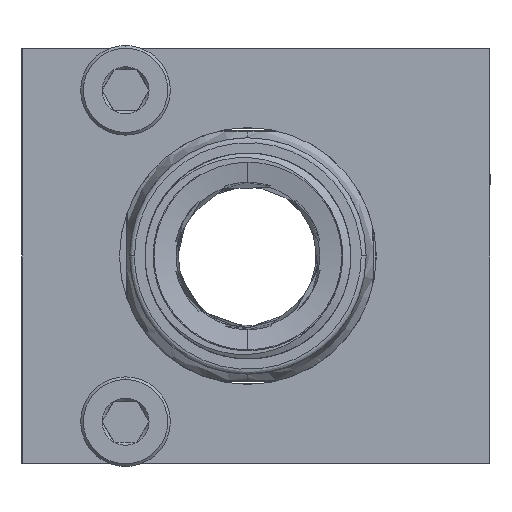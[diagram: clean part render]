
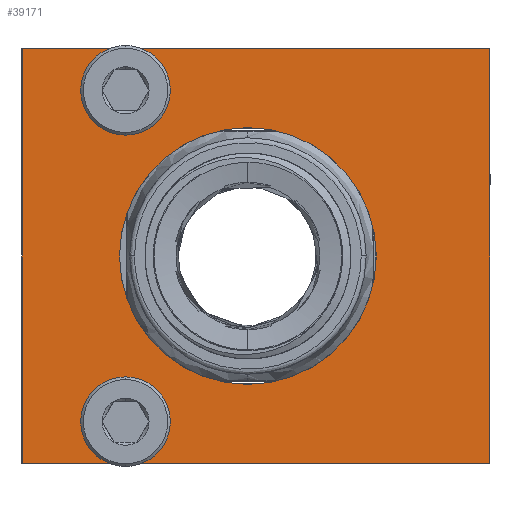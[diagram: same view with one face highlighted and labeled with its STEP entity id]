
A CAD part, left-side view. The second image highlights one B-rep face of the part: STEP entity #39171.
In plain terms, the highlighted face is planar.
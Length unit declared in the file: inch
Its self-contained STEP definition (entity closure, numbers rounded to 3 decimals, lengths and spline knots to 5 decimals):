
#398 = CARTESIAN_POINT ( 'NONE',  ( 0.1, -0.25, 0. ) ) ;
#2111 = CIRCLE ( 'NONE', #46787, 0.06693 ) ;
#2180 = CARTESIAN_POINT ( 'NONE',  ( 0., 0., 0. ) ) ;
#2478 = CARTESIAN_POINT ( 'NONE',  ( 0., -1.13, 0. ) ) ;
#2892 = CARTESIAN_POINT ( 'NONE',  ( 0.83307, -0.25, 0. ) ) ;
#3965 = CARTESIAN_POINT ( 'NONE',  ( 0., 0., 0. ) ) ;
#5410 = CARTESIAN_POINT ( 'NONE',  ( 0.03307, -0.25, 0. ) ) ;
#6128 = ORIENTED_EDGE ( 'NONE', *, *, #40474, .F. ) ;
#6226 = CARTESIAN_POINT ( 'NONE',  ( 1., 0., 0. ) ) ;
#8245 = VERTEX_POINT ( 'NONE', #2478 ) ;
#8386 = DIRECTION ( 'NONE',  ( 1., 0., 0. ) ) ;
#8398 = LINE ( 'NONE', #37738, #50243 ) ;
#8513 = CIRCLE ( 'NONE', #46215, 0.31 ) ;
#8878 = ORIENTED_EDGE ( 'NONE', *, *, #20147, .F. ) ;
#9260 = CARTESIAN_POINT ( 'NONE',  ( 0., -1.13, 0. ) ) ;
#9750 = CIRCLE ( 'NONE', #53628, 0.06693 ) ;
#10035 = VERTEX_POINT ( 'NONE', #11764 ) ;
#11414 = CARTESIAN_POINT ( 'NONE',  ( 0.5, -0.5454, 0. ) ) ;
#11764 = CARTESIAN_POINT ( 'NONE',  ( 0.19, -0.5454, 0. ) ) ;
#12238 = DIRECTION ( 'NONE',  ( 0., 0., 1. ) ) ;
#13380 = EDGE_CURVE ( 'NONE', #33789, #44122, #49512, .T. ) ;
#13901 = CARTESIAN_POINT ( 'NONE',  ( 0., 0., 0. ) ) ;
#14447 = LINE ( 'NONE', #13901, #34724 ) ;
#16477 = CARTESIAN_POINT ( 'NONE',  ( 0.9, -0.25, 0. ) ) ;
#16514 = ORIENTED_EDGE ( 'NONE', *, *, #27187, .F. ) ;
#16700 = ORIENTED_EDGE ( 'NONE', *, *, #13380, .T. ) ;
#17925 = EDGE_LOOP ( 'NONE', ( #16514, #19743, #43461, #8878 ) ) ;
#18014 = EDGE_CURVE ( 'NONE', #28951, #38390, #35108, .T. ) ;
#19743 = ORIENTED_EDGE ( 'NONE', *, *, #47596, .F. ) ;
#20147 = EDGE_CURVE ( 'NONE', #8245, #36006, #42175, .T. ) ;
#20485 = VERTEX_POINT ( 'NONE', #34172 ) ;
#20861 = DIRECTION ( 'NONE',  ( 1., 0., 0. ) ) ;
#20984 = LINE ( 'NONE', #3965, #35460 ) ;
#21788 = EDGE_CURVE ( 'NONE', #38390, #28951, #9750, .T. ) ;
#22515 = CARTESIAN_POINT ( 'NONE',  ( 0.96693, -0.25, 0. ) ) ;
#22802 = DIRECTION ( 'NONE',  ( 0., 0., 1. ) ) ;
#22865 = EDGE_LOOP ( 'NONE', ( #30108, #6128 ) ) ;
#23784 = EDGE_CURVE ( 'NONE', #10035, #20485, #24668, .T. ) ;
#24280 = DIRECTION ( 'NONE',  ( -1., 0., 0. ) ) ;
#24401 = DIRECTION ( 'NONE',  ( 1., 0., 0. ) ) ;
#24527 = DIRECTION ( 'NONE',  ( 0., 0., -1. ) ) ;
#24668 = CIRCLE ( 'NONE', #46636, 0.31 ) ;
#24813 = DIRECTION ( 'NONE',  ( 0., -1., 0. ) ) ;
#24958 = DIRECTION ( 'NONE',  ( 0., 0., 1. ) ) ;
#26301 = EDGE_LOOP ( 'NONE', ( #39288, #43027 ) ) ;
#26504 = DIRECTION ( 'NONE',  ( -1., 0., 0. ) ) ;
#26770 = ORIENTED_EDGE ( 'NONE', *, *, #35489, .T. ) ;
#27187 = EDGE_CURVE ( 'NONE', #44794, #8245, #20984, .T. ) ;
#27195 = DIRECTION ( 'NONE',  ( 1., 0., 0. ) ) ;
#28117 = CARTESIAN_POINT ( 'NONE',  ( 0.5, -0.5454, 0. ) ) ;
#28908 = DIRECTION ( 'NONE',  ( -1., 0., 0. ) ) ;
#28951 = VERTEX_POINT ( 'NONE', #45746 ) ;
#29772 = FACE_OUTER_BOUND ( 'NONE', #17925, .T. ) ;
#30108 = ORIENTED_EDGE ( 'NONE', *, *, #23784, .F. ) ;
#32646 = DIRECTION ( 'NONE',  ( 0., 0., 1. ) ) ;
#33095 = PLANE ( 'NONE',  #47887 ) ;
#33789 = VERTEX_POINT ( 'NONE', #2892 ) ;
#33929 = FACE_BOUND ( 'NONE', #22865, .T. ) ;
#33950 = EDGE_LOOP ( 'NONE', ( #26770, #16700 ) ) ;
#34172 = CARTESIAN_POINT ( 'NONE',  ( 0.81, -0.5454, 0. ) ) ;
#34724 = VECTOR ( 'NONE', #26504, 39.37008 ) ;
#34891 = CARTESIAN_POINT ( 'NONE',  ( 0.9, -0.25, 0. ) ) ;
#35108 = CIRCLE ( 'NONE', #40335, 0.06693 ) ;
#35460 = VECTOR ( 'NONE', #24813, 39.37008 ) ;
#35489 = EDGE_CURVE ( 'NONE', #44122, #33789, #2111, .T. ) ;
#36006 = VERTEX_POINT ( 'NONE', #52572 ) ;
#36750 = CARTESIAN_POINT ( 'NONE',  ( 0.1, -0.25, 0. ) ) ;
#37277 = VECTOR ( 'NONE', #38052, 39.37008 ) ;
#37738 = CARTESIAN_POINT ( 'NONE',  ( 1., 0., 0. ) ) ;
#38052 = DIRECTION ( 'NONE',  ( 1., 0., 0. ) ) ;
#38390 = VERTEX_POINT ( 'NONE', #5410 ) ;
#38787 = DIRECTION ( 'NONE',  ( 1., 0., 0. ) ) ;
#39058 = VERTEX_POINT ( 'NONE', #6226 ) ;
#39171 = ADVANCED_FACE ( 'NONE', ( #33929, #50660, #46000, #29772 ), #33095, .F. ) ;
#39288 = ORIENTED_EDGE ( 'NONE', *, *, #18014, .T. ) ;
#40335 = AXIS2_PLACEMENT_3D ( 'NONE', #398, #42667, #8386 ) ;
#40474 = EDGE_CURVE ( 'NONE', #20485, #10035, #8513, .T. ) ;
#42175 = LINE ( 'NONE', #9260, #37277 ) ;
#42667 = DIRECTION ( 'NONE',  ( 0., 0., 1. ) ) ;
#42680 = DIRECTION ( 'NONE',  ( 0., 1., 0. ) ) ;
#43027 = ORIENTED_EDGE ( 'NONE', *, *, #21788, .T. ) ;
#43461 = ORIENTED_EDGE ( 'NONE', *, *, #47283, .F. ) ;
#44122 = VERTEX_POINT ( 'NONE', #22515 ) ;
#44794 = VERTEX_POINT ( 'NONE', #2180 ) ;
#45746 = CARTESIAN_POINT ( 'NONE',  ( 0.16693, -0.25, 0. ) ) ;
#46000 = FACE_BOUND ( 'NONE', #33950, .T. ) ;
#46215 = AXIS2_PLACEMENT_3D ( 'NONE', #11414, #53671, #24280 ) ;
#46636 = AXIS2_PLACEMENT_3D ( 'NONE', #28117, #24527, #28908 ) ;
#46787 = AXIS2_PLACEMENT_3D ( 'NONE', #34891, #22802, #27195 ) ;
#47283 = EDGE_CURVE ( 'NONE', #36006, #39058, #8398, .T. ) ;
#47596 = EDGE_CURVE ( 'NONE', #39058, #44794, #14447, .T. ) ;
#47876 = AXIS2_PLACEMENT_3D ( 'NONE', #16477, #24958, #20861 ) ;
#47887 = AXIS2_PLACEMENT_3D ( 'NONE', #49846, #12238, #38787 ) ;
#49512 = CIRCLE ( 'NONE', #47876, 0.06693 ) ;
#49846 = CARTESIAN_POINT ( 'NONE',  ( 0., 0., 0. ) ) ;
#50243 = VECTOR ( 'NONE', #42680, 39.37008 ) ;
#50660 = FACE_BOUND ( 'NONE', #26301, .T. ) ;
#52572 = CARTESIAN_POINT ( 'NONE',  ( 1., -1.13, 0. ) ) ;
#53628 = AXIS2_PLACEMENT_3D ( 'NONE', #36750, #32646, #24401 ) ;
#53671 = DIRECTION ( 'NONE',  ( 0., 0., -1. ) ) ;
